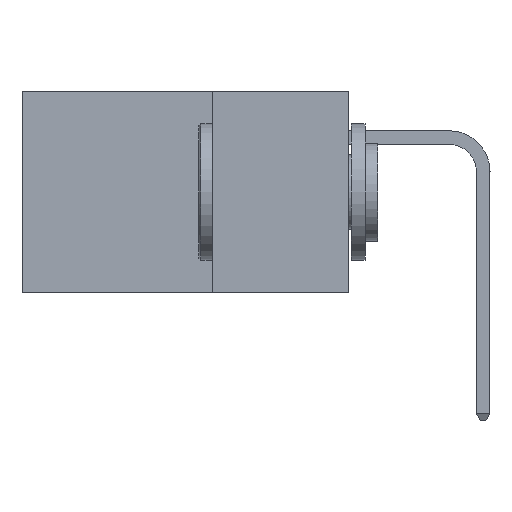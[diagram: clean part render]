
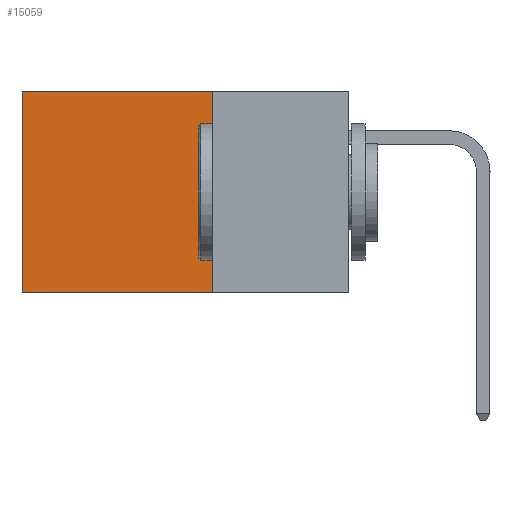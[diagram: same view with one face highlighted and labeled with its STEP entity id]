
A CAD part, left-side view. The second image highlights one B-rep face of the part: STEP entity #15059.
In plain terms, the highlighted planar face has unit normal (-1, 0, 0).
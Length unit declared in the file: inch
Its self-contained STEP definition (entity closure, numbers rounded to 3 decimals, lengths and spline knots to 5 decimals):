
#370 = VERTEX_POINT ( 'NONE', #12680 ) ;
#533 = VERTEX_POINT ( 'NONE', #3511 ) ;
#589 = VECTOR ( 'NONE', #37799, 39.37008 ) ;
#1391 = DIRECTION ( 'NONE',  ( 0., 1., 0. ) ) ;
#1411 = LINE ( 'NONE', #30582, #6888 ) ;
#2143 = LINE ( 'NONE', #8239, #38297 ) ;
#2764 = CARTESIAN_POINT ( 'NONE',  ( 0.2875, 0.25, 0. ) ) ;
#3511 = CARTESIAN_POINT ( 'NONE',  ( 0.2875, 0.25, 0. ) ) ;
#5225 = ORIENTED_EDGE ( 'NONE', *, *, #28184, .F. ) ;
#5767 = VECTOR ( 'NONE', #11688, 39.37008 ) ;
#6888 = VECTOR ( 'NONE', #1391, 39.37008 ) ;
#7983 = CARTESIAN_POINT ( 'NONE',  ( 0.2875, 0.6, -0.37 ) ) ;
#8239 = CARTESIAN_POINT ( 'NONE',  ( 0.2875, 0.25, 0. ) ) ;
#11688 = DIRECTION ( 'NONE',  ( 0., 0., -1. ) ) ;
#12450 = PLANE ( 'NONE',  #35928 ) ;
#12680 = CARTESIAN_POINT ( 'NONE',  ( 0.2875, 0.25, -0.37 ) ) ;
#12715 = VERTEX_POINT ( 'NONE', #30398 ) ;
#13563 = EDGE_CURVE ( 'NONE', #533, #12715, #1411, .T. ) ;
#14732 = DIRECTION ( 'NONE',  ( 0., 0., -1. ) ) ;
#15059 = ADVANCED_FACE ( 'NONE', ( #18876 ), #12450, .F. ) ;
#16620 = EDGE_CURVE ( 'NONE', #370, #26230, #34748, .T. ) ;
#18293 = CARTESIAN_POINT ( 'NONE',  ( 0.2875, 0.6, 0. ) ) ;
#18876 = FACE_OUTER_BOUND ( 'NONE', #22091, .T. ) ;
#19812 = LINE ( 'NONE', #18293, #5767 ) ;
#21075 = EDGE_CURVE ( 'NONE', #12715, #26230, #19812, .T. ) ;
#22091 = EDGE_LOOP ( 'NONE', ( #31451, #25285, #5225, #38995 ) ) ;
#25285 = ORIENTED_EDGE ( 'NONE', *, *, #16620, .F. ) ;
#26230 = VERTEX_POINT ( 'NONE', #7983 ) ;
#28184 = EDGE_CURVE ( 'NONE', #533, #370, #2143, .T. ) ;
#29264 = DIRECTION ( 'NONE',  ( 0., 0., -1. ) ) ;
#30398 = CARTESIAN_POINT ( 'NONE',  ( 0.2875, 0.6, 0. ) ) ;
#30582 = CARTESIAN_POINT ( 'NONE',  ( 0.2875, 0.25, 0. ) ) ;
#31451 = ORIENTED_EDGE ( 'NONE', *, *, #21075, .T. ) ;
#34748 = LINE ( 'NONE', #35407, #589 ) ;
#35407 = CARTESIAN_POINT ( 'NONE',  ( 0.2875, 0.25, -0.37 ) ) ;
#35928 = AXIS2_PLACEMENT_3D ( 'NONE', #2764, #41097, #29264 ) ;
#37799 = DIRECTION ( 'NONE',  ( 0., 1., 0. ) ) ;
#38297 = VECTOR ( 'NONE', #14732, 39.37008 ) ;
#38995 = ORIENTED_EDGE ( 'NONE', *, *, #13563, .T. ) ;
#41097 = DIRECTION ( 'NONE',  ( 1., 0., 0. ) ) ;
